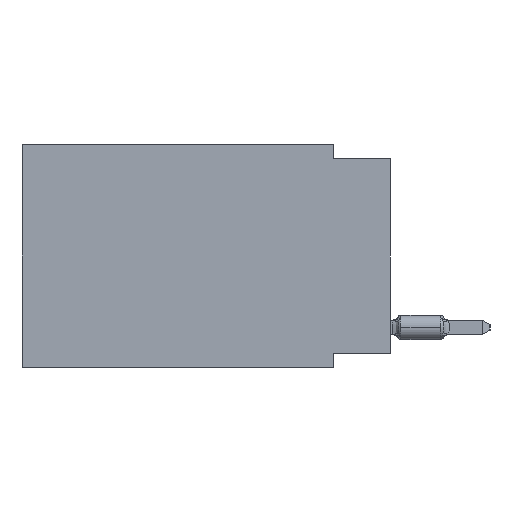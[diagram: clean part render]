
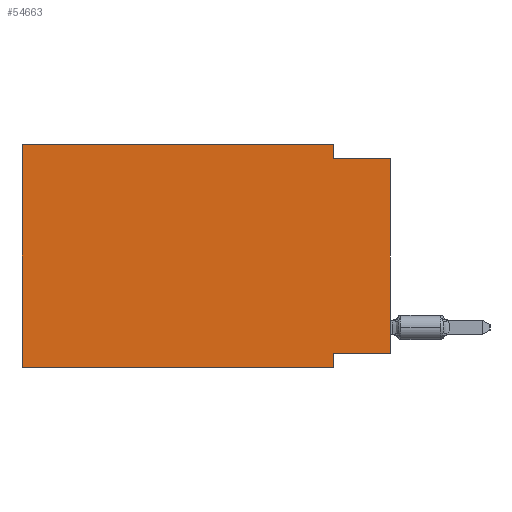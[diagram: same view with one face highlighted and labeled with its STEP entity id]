
A CAD part, left-side view. The second image highlights one B-rep face of the part: STEP entity #54663.
In plain terms, the highlighted planar face has unit normal (-1, 0, 0).
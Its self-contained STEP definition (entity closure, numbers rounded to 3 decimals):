
#444 = EDGE_CURVE ( 'NONE', #49894, #10901, #19748, .T. ) ;
#1547 = CARTESIAN_POINT ( 'NONE',  ( 0., 0., -0.635 ) ) ;
#2123 = AXIS2_PLACEMENT_3D ( 'NONE', #6908, #27525, #23257 ) ;
#2958 = EDGE_LOOP ( 'NONE', ( #34275, #31388, #28525, #60935, #9429, #62071, #40463, #11947 ) ) ;
#3004 = DIRECTION ( 'NONE',  ( 0., 0., -1. ) ) ;
#3341 = VECTOR ( 'NONE', #19061, 1000. ) ;
#5240 = CARTESIAN_POINT ( 'NONE',  ( 0., 2.54, -9.906 ) ) ;
#6630 = CARTESIAN_POINT ( 'NONE',  ( 0., 2.54, -9.271 ) ) ;
#6908 = CARTESIAN_POINT ( 'NONE',  ( 0., 16.383, 0. ) ) ;
#8590 = LINE ( 'NONE', #19699, #3341 ) ;
#8656 = DIRECTION ( 'NONE',  ( 0., 0., 1. ) ) ;
#9429 = ORIENTED_EDGE ( 'NONE', *, *, #32690, .F. ) ;
#9914 = CARTESIAN_POINT ( 'NONE',  ( 0., 0., -9.271 ) ) ;
#10187 = DIRECTION ( 'NONE',  ( 0., 0., -1. ) ) ;
#10235 = CARTESIAN_POINT ( 'NONE',  ( 0., 0., 0. ) ) ;
#10237 = DIRECTION ( 'NONE',  ( 0., -1., 0. ) ) ;
#10635 = VECTOR ( 'NONE', #44677, 1000. ) ;
#10901 = VERTEX_POINT ( 'NONE', #5240 ) ;
#11947 = ORIENTED_EDGE ( 'NONE', *, *, #16510, .F. ) ;
#13189 = CARTESIAN_POINT ( 'NONE',  ( 0., 16.383, 0. ) ) ;
#13228 = CARTESIAN_POINT ( 'NONE',  ( 0., 16.383, 0. ) ) ;
#14824 = EDGE_CURVE ( 'NONE', #63788, #49596, #60063, .T. ) ;
#16510 = EDGE_CURVE ( 'NONE', #54726, #53007, #43682, .T. ) ;
#16580 = EDGE_CURVE ( 'NONE', #54726, #39270, #55454, .T. ) ;
#18819 = VECTOR ( 'NONE', #3004, 1000. ) ;
#19061 = DIRECTION ( 'NONE',  ( 0., -1., 0. ) ) ;
#19395 = EDGE_CURVE ( 'NONE', #62379, #39270, #8590, .T. ) ;
#19699 = CARTESIAN_POINT ( 'NONE',  ( 0., 0., -0.635 ) ) ;
#19748 = LINE ( 'NONE', #31428, #10635 ) ;
#23257 = DIRECTION ( 'NONE',  ( 0., 0., -1. ) ) ;
#24212 = VECTOR ( 'NONE', #8656, 1000. ) ;
#27525 = DIRECTION ( 'NONE',  ( 1., 0., 0. ) ) ;
#28175 = FACE_OUTER_BOUND ( 'NONE', #2958, .T. ) ;
#28525 = ORIENTED_EDGE ( 'NONE', *, *, #31149, .F. ) ;
#31149 = EDGE_CURVE ( 'NONE', #49596, #62379, #32806, .T. ) ;
#31388 = ORIENTED_EDGE ( 'NONE', *, *, #19395, .F. ) ;
#31428 = CARTESIAN_POINT ( 'NONE',  ( 0., 16.383, -9.906 ) ) ;
#32690 = EDGE_CURVE ( 'NONE', #49894, #63788, #64373, .T. ) ;
#32806 = LINE ( 'NONE', #38383, #18819 ) ;
#34275 = ORIENTED_EDGE ( 'NONE', *, *, #16580, .T. ) ;
#35428 = CARTESIAN_POINT ( 'NONE',  ( 0., 2.54, -0.635 ) ) ;
#36085 = DIRECTION ( 'NONE',  ( 0., 0., 1. ) ) ;
#36731 = CARTESIAN_POINT ( 'NONE',  ( 0., 0., -9.271 ) ) ;
#38383 = CARTESIAN_POINT ( 'NONE',  ( 0., 2.54, 0. ) ) ;
#39270 = VERTEX_POINT ( 'NONE', #1547 ) ;
#39422 = CARTESIAN_POINT ( 'NONE',  ( 0., 16.383, 0. ) ) ;
#40017 = CARTESIAN_POINT ( 'NONE',  ( 0., 2.54, -9.906 ) ) ;
#40463 = ORIENTED_EDGE ( 'NONE', *, *, #41138, .F. ) ;
#41138 = EDGE_CURVE ( 'NONE', #53007, #10901, #56042, .T. ) ;
#43681 = CARTESIAN_POINT ( 'NONE',  ( 0., 2.54, 0. ) ) ;
#43682 = LINE ( 'NONE', #9914, #51260 ) ;
#44677 = DIRECTION ( 'NONE',  ( 0., -1., 0. ) ) ;
#47861 = CARTESIAN_POINT ( 'NONE',  ( 0., 16.383, -9.906 ) ) ;
#49596 = VERTEX_POINT ( 'NONE', #43681 ) ;
#49894 = VERTEX_POINT ( 'NONE', #47861 ) ;
#51260 = VECTOR ( 'NONE', #58426, 1000. ) ;
#52202 = VECTOR ( 'NONE', #10237, 1000. ) ;
#53007 = VERTEX_POINT ( 'NONE', #6630 ) ;
#54663 = ADVANCED_FACE ( 'NONE', ( #28175 ), #57999, .F. ) ;
#54726 = VERTEX_POINT ( 'NONE', #36731 ) ;
#55454 = LINE ( 'NONE', #10235, #59629 ) ;
#56042 = LINE ( 'NONE', #40017, #57236 ) ;
#57236 = VECTOR ( 'NONE', #10187, 1000. ) ;
#57999 = PLANE ( 'NONE',  #2123 ) ;
#58426 = DIRECTION ( 'NONE',  ( 0., 1., 0. ) ) ;
#59629 = VECTOR ( 'NONE', #36085, 1000. ) ;
#60063 = LINE ( 'NONE', #39422, #52202 ) ;
#60935 = ORIENTED_EDGE ( 'NONE', *, *, #14824, .F. ) ;
#62071 = ORIENTED_EDGE ( 'NONE', *, *, #444, .T. ) ;
#62379 = VERTEX_POINT ( 'NONE', #35428 ) ;
#63788 = VERTEX_POINT ( 'NONE', #13189 ) ;
#64373 = LINE ( 'NONE', #13228, #24212 ) ;
